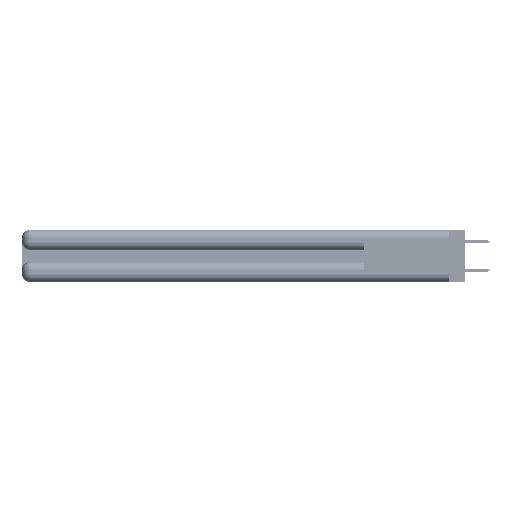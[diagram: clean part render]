
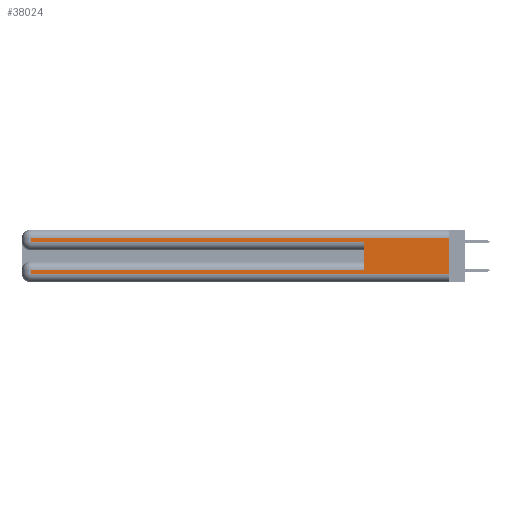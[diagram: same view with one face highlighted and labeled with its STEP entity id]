
A CAD part, left-side view. The second image highlights one B-rep face of the part: STEP entity #38024.
In plain terms, the highlighted planar face has unit normal (-1, 0, 0).
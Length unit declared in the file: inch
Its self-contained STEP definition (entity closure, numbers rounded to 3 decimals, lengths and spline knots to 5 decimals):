
#788 = LINE ( 'NONE', #14265, #23515 ) ;
#1238 = LINE ( 'NONE', #35794, #52657 ) ;
#1759 = ORIENTED_EDGE ( 'NONE', *, *, #52632, .T. ) ;
#2255 = ORIENTED_EDGE ( 'NONE', *, *, #34191, .T. ) ;
#4033 = VECTOR ( 'NONE', #41554, 39.37008 ) ;
#4771 = PLANE ( 'NONE',  #25293 ) ;
#5344 = DIRECTION ( 'NONE',  ( 0., 1., 0. ) ) ;
#6481 = VERTEX_POINT ( 'NONE', #7855 ) ;
#6992 = CARTESIAN_POINT ( 'NONE',  ( 0., 2.94, 0.06 ) ) ;
#7855 = CARTESIAN_POINT ( 'NONE',  ( 0., 0.6, 0.285 ) ) ;
#8625 = LINE ( 'NONE', #22347, #27318 ) ;
#9981 = DIRECTION ( 'NONE',  ( 0., 0., -1. ) ) ;
#14265 = CARTESIAN_POINT ( 'NONE',  ( 0., 2.94, 0.37 ) ) ;
#14324 = EDGE_CURVE ( 'NONE', #33664, #52515, #8625, .T. ) ;
#14414 = EDGE_CURVE ( 'NONE', #33664, #27822, #1238, .T. ) ;
#14864 = VERTEX_POINT ( 'NONE', #42824 ) ;
#15433 = LINE ( 'NONE', #26520, #36199 ) ;
#20505 = DIRECTION ( 'NONE',  ( 0., -1., 0. ) ) ;
#21862 = DIRECTION ( 'NONE',  ( 0., 1., 0. ) ) ;
#21965 = DIRECTION ( 'NONE',  ( 0., 0., -1. ) ) ;
#22347 = CARTESIAN_POINT ( 'NONE',  ( 0., 0., 0.31 ) ) ;
#23515 = VECTOR ( 'NONE', #9981, 39.37008 ) ;
#24025 = CARTESIAN_POINT ( 'NONE',  ( 0., 2.94, 0.31 ) ) ;
#24357 = LINE ( 'NONE', #34854, #35675 ) ;
#25026 = ORIENTED_EDGE ( 'NONE', *, *, #36598, .F. ) ;
#25293 = AXIS2_PLACEMENT_3D ( 'NONE', #34663, #25698, #21965 ) ;
#25642 = VECTOR ( 'NONE', #20505, 39.37008 ) ;
#25698 = DIRECTION ( 'NONE',  ( 1., 0., 0. ) ) ;
#25886 = VERTEX_POINT ( 'NONE', #52425 ) ;
#25957 = EDGE_LOOP ( 'NONE', ( #41133, #43733, #53135, #1759, #25026, #30207, #36125, #2255 ) ) ;
#26520 = CARTESIAN_POINT ( 'NONE',  ( 0., 0., 0.085 ) ) ;
#27318 = VECTOR ( 'NONE', #5344, 39.37008 ) ;
#27822 = VERTEX_POINT ( 'NONE', #52623 ) ;
#28340 = LINE ( 'NONE', #42184, #25642 ) ;
#30207 = ORIENTED_EDGE ( 'NONE', *, *, #44309, .T. ) ;
#31311 = VERTEX_POINT ( 'NONE', #6992 ) ;
#33664 = VERTEX_POINT ( 'NONE', #49172 ) ;
#34191 = EDGE_CURVE ( 'NONE', #31311, #27822, #28340, .T. ) ;
#34663 = CARTESIAN_POINT ( 'NONE',  ( 0., 0., 0.37 ) ) ;
#34854 = CARTESIAN_POINT ( 'NONE',  ( 0., 0.6, 0.145 ) ) ;
#35255 = EDGE_CURVE ( 'NONE', #52515, #25886, #788, .T. ) ;
#35675 = VECTOR ( 'NONE', #52399, 39.37008 ) ;
#35794 = CARTESIAN_POINT ( 'NONE',  ( 0., 0., 0.37 ) ) ;
#36125 = ORIENTED_EDGE ( 'NONE', *, *, #48894, .T. ) ;
#36199 = VECTOR ( 'NONE', #21862, 39.37008 ) ;
#36598 = EDGE_CURVE ( 'NONE', #53044, #6481, #24357, .T. ) ;
#38024 = ADVANCED_FACE ( 'NONE', ( #50178 ), #4771, .F. ) ;
#40997 = CARTESIAN_POINT ( 'NONE',  ( 0., 2.94, 0.37 ) ) ;
#41061 = LINE ( 'NONE', #40997, #51072 ) ;
#41133 = ORIENTED_EDGE ( 'NONE', *, *, #14414, .F. ) ;
#41554 = DIRECTION ( 'NONE',  ( 0., -1., 0. ) ) ;
#42184 = CARTESIAN_POINT ( 'NONE',  ( 0., 0., 0.06 ) ) ;
#42824 = CARTESIAN_POINT ( 'NONE',  ( 0., 2.94, 0.085 ) ) ;
#43733 = ORIENTED_EDGE ( 'NONE', *, *, #14324, .T. ) ;
#44309 = EDGE_CURVE ( 'NONE', #53044, #14864, #15433, .T. ) ;
#45374 = CARTESIAN_POINT ( 'NONE',  ( 0., 0.6, 0.085 ) ) ;
#48690 = DIRECTION ( 'NONE',  ( 0., 0., -1. ) ) ;
#48894 = EDGE_CURVE ( 'NONE', #14864, #31311, #41061, .T. ) ;
#49172 = CARTESIAN_POINT ( 'NONE',  ( 0., 0., 0.31 ) ) ;
#49426 = DIRECTION ( 'NONE',  ( 0., 0., -1. ) ) ;
#49440 = CARTESIAN_POINT ( 'NONE',  ( 0., 0., 0.285 ) ) ;
#50178 = FACE_OUTER_BOUND ( 'NONE', #25957, .T. ) ;
#51072 = VECTOR ( 'NONE', #49426, 39.37008 ) ;
#52147 = LINE ( 'NONE', #49440, #4033 ) ;
#52399 = DIRECTION ( 'NONE',  ( 0., 0., 1. ) ) ;
#52425 = CARTESIAN_POINT ( 'NONE',  ( 0., 2.94, 0.285 ) ) ;
#52515 = VERTEX_POINT ( 'NONE', #24025 ) ;
#52623 = CARTESIAN_POINT ( 'NONE',  ( 0., 0., 0.06 ) ) ;
#52632 = EDGE_CURVE ( 'NONE', #25886, #6481, #52147, .T. ) ;
#52657 = VECTOR ( 'NONE', #48690, 39.37008 ) ;
#53044 = VERTEX_POINT ( 'NONE', #45374 ) ;
#53135 = ORIENTED_EDGE ( 'NONE', *, *, #35255, .T. ) ;
